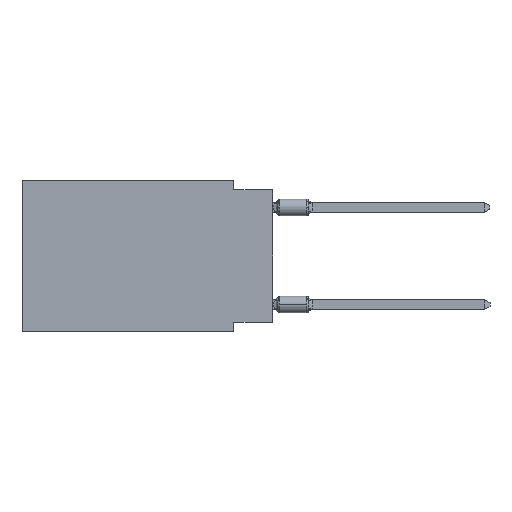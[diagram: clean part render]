
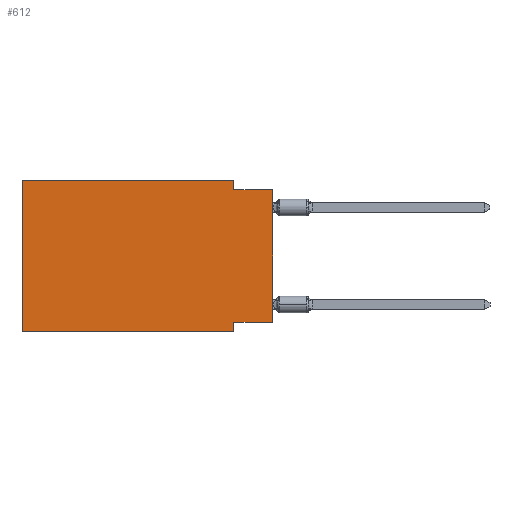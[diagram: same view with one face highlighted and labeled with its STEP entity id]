
A CAD part, left-side view. The second image highlights one B-rep face of the part: STEP entity #612.
In plain terms, the highlighted planar face has unit normal (-1, 0, 0).
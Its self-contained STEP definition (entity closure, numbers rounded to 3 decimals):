
#518 = CARTESIAN_POINT ( 'NONE',  ( 0., 16.383, 0. ) ) ;
#612 = ADVANCED_FACE ( 'NONE', ( #7089 ), #5715, .F. ) ;
#798 = ORIENTED_EDGE ( 'NONE', *, *, #16910, .F. ) ;
#809 = DIRECTION ( 'NONE',  ( 0., 0., 1. ) ) ;
#1196 = DIRECTION ( 'NONE',  ( 0., 0., -1. ) ) ;
#1422 = CARTESIAN_POINT ( 'NONE',  ( 0., 0., -9.271 ) ) ;
#1513 = ORIENTED_EDGE ( 'NONE', *, *, #11905, .F. ) ;
#1604 = CARTESIAN_POINT ( 'NONE',  ( 0., 2.54, -9.906 ) ) ;
#1825 = CARTESIAN_POINT ( 'NONE',  ( 0., 0., -0.635 ) ) ;
#2154 = EDGE_CURVE ( 'NONE', #9533, #7380, #8612, .T. ) ;
#2157 = DIRECTION ( 'NONE',  ( 0., 1., 0. ) ) ;
#2253 = CARTESIAN_POINT ( 'NONE',  ( 0., 16.383, -9.906 ) ) ;
#2658 = VERTEX_POINT ( 'NONE', #3082 ) ;
#2768 = ORIENTED_EDGE ( 'NONE', *, *, #13945, .F. ) ;
#2803 = CARTESIAN_POINT ( 'NONE',  ( 0., 16.383, 0. ) ) ;
#3082 = CARTESIAN_POINT ( 'NONE',  ( 0., 2.54, -0.635 ) ) ;
#3514 = ORIENTED_EDGE ( 'NONE', *, *, #6840, .T. ) ;
#3604 = DIRECTION ( 'NONE',  ( 0., -1., 0. ) ) ;
#3798 = LINE ( 'NONE', #10373, #10157 ) ;
#3864 = CARTESIAN_POINT ( 'NONE',  ( 0., 16.383, -9.906 ) ) ;
#3882 = VECTOR ( 'NONE', #13414, 1000. ) ;
#4088 = CARTESIAN_POINT ( 'NONE',  ( 0., 0., -9.271 ) ) ;
#4382 = CARTESIAN_POINT ( 'NONE',  ( 0., 0., -0.635 ) ) ;
#4463 = VECTOR ( 'NONE', #3604, 1000. ) ;
#4486 = CARTESIAN_POINT ( 'NONE',  ( 0., 2.54, -9.271 ) ) ;
#4627 = LINE ( 'NONE', #7113, #11128 ) ;
#4787 = VECTOR ( 'NONE', #5581, 1000. ) ;
#5043 = EDGE_CURVE ( 'NONE', #9533, #16462, #11977, .T. ) ;
#5332 = ORIENTED_EDGE ( 'NONE', *, *, #8408, .F. ) ;
#5532 = VERTEX_POINT ( 'NONE', #2803 ) ;
#5581 = DIRECTION ( 'NONE',  ( 0., -1., 0. ) ) ;
#5715 = PLANE ( 'NONE',  #11506 ) ;
#5798 = DIRECTION ( 'NONE',  ( 0., 0., -1. ) ) ;
#6033 = CARTESIAN_POINT ( 'NONE',  ( 0., 0., 0. ) ) ;
#6778 = LINE ( 'NONE', #1604, #3882 ) ;
#6840 = EDGE_CURVE ( 'NONE', #11544, #14137, #14117, .T. ) ;
#7089 = FACE_OUTER_BOUND ( 'NONE', #15639, .T. ) ;
#7108 = VECTOR ( 'NONE', #1196, 1000. ) ;
#7113 = CARTESIAN_POINT ( 'NONE',  ( 0., 16.383, 0. ) ) ;
#7380 = VERTEX_POINT ( 'NONE', #1825 ) ;
#7533 = CARTESIAN_POINT ( 'NONE',  ( 0., 2.54, 0. ) ) ;
#7745 = LINE ( 'NONE', #13094, #7108 ) ;
#8273 = DIRECTION ( 'NONE',  ( 0., 0., 1. ) ) ;
#8408 = EDGE_CURVE ( 'NONE', #11544, #5532, #4627, .T. ) ;
#8612 = LINE ( 'NONE', #6033, #12398 ) ;
#9533 = VERTEX_POINT ( 'NONE', #1422 ) ;
#9545 = EDGE_CURVE ( 'NONE', #16462, #14137, #6778, .T. ) ;
#10157 = VECTOR ( 'NONE', #12833, 1000. ) ;
#10373 = CARTESIAN_POINT ( 'NONE',  ( 0., 16.383, 0. ) ) ;
#10865 = ORIENTED_EDGE ( 'NONE', *, *, #9545, .F. ) ;
#10890 = CARTESIAN_POINT ( 'NONE',  ( 0., 2.54, -9.906 ) ) ;
#11128 = VECTOR ( 'NONE', #809, 1000. ) ;
#11471 = VECTOR ( 'NONE', #2157, 1000. ) ;
#11506 = AXIS2_PLACEMENT_3D ( 'NONE', #518, #13818, #5798 ) ;
#11544 = VERTEX_POINT ( 'NONE', #2253 ) ;
#11905 = EDGE_CURVE ( 'NONE', #16949, #2658, #7745, .T. ) ;
#11977 = LINE ( 'NONE', #4088, #11471 ) ;
#12398 = VECTOR ( 'NONE', #8273, 1000. ) ;
#12833 = DIRECTION ( 'NONE',  ( 0., -1., 0. ) ) ;
#13094 = CARTESIAN_POINT ( 'NONE',  ( 0., 2.54, 0. ) ) ;
#13414 = DIRECTION ( 'NONE',  ( 0., 0., -1. ) ) ;
#13818 = DIRECTION ( 'NONE',  ( 1., 0., 0. ) ) ;
#13945 = EDGE_CURVE ( 'NONE', #5532, #16949, #3798, .T. ) ;
#14117 = LINE ( 'NONE', #3864, #4463 ) ;
#14137 = VERTEX_POINT ( 'NONE', #10890 ) ;
#14181 = ORIENTED_EDGE ( 'NONE', *, *, #5043, .F. ) ;
#14550 = ORIENTED_EDGE ( 'NONE', *, *, #2154, .T. ) ;
#15639 = EDGE_LOOP ( 'NONE', ( #14550, #798, #1513, #2768, #5332, #3514, #10865, #14181 ) ) ;
#16269 = LINE ( 'NONE', #4382, #4787 ) ;
#16462 = VERTEX_POINT ( 'NONE', #4486 ) ;
#16910 = EDGE_CURVE ( 'NONE', #2658, #7380, #16269, .T. ) ;
#16949 = VERTEX_POINT ( 'NONE', #7533 ) ;
